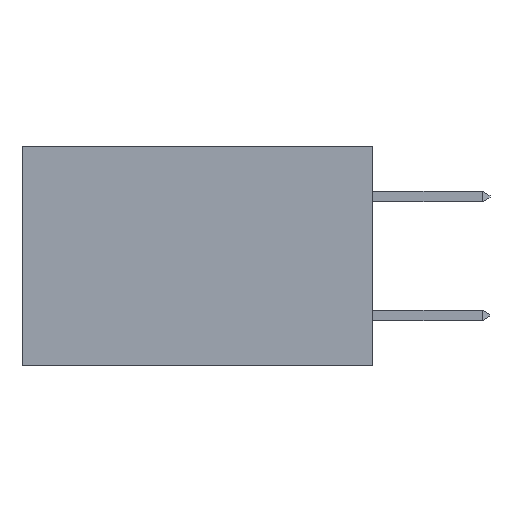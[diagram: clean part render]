
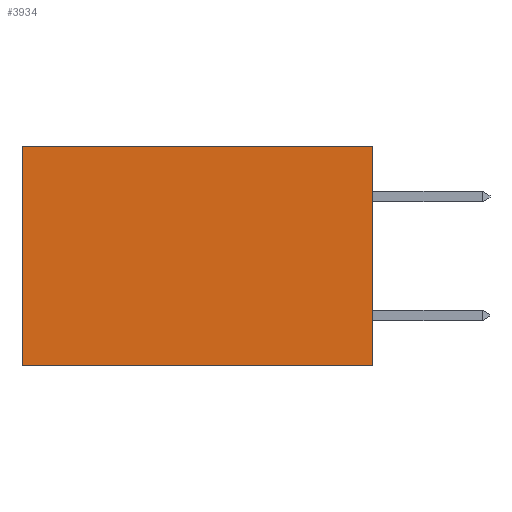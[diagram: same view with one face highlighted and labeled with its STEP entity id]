
A CAD part, left-side view. The second image highlights one B-rep face of the part: STEP entity #3934.
In plain terms, the highlighted planar face has unit normal (-1, 0, 0).
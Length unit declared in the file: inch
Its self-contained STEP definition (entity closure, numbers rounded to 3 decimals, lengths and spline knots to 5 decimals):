
#102 = ORIENTED_EDGE ( 'NONE', *, *, #2369, .F. ) ;
#112 = ORIENTED_EDGE ( 'NONE', *, *, #5296, .F. ) ;
#225 = CARTESIAN_POINT ( 'NONE',  ( 0.277, 0., 0. ) ) ;
#416 = DIRECTION ( 'NONE',  ( 0., 0., -1. ) ) ;
#442 = DIRECTION ( 'NONE',  ( 1., 0., 0. ) ) ;
#554 = CARTESIAN_POINT ( 'NONE',  ( 0.277, 0., -0.37 ) ) ;
#694 = EDGE_CURVE ( 'NONE', #3943, #6967, #5586, .T. ) ;
#910 = VERTEX_POINT ( 'NONE', #6572 ) ;
#919 = AXIS2_PLACEMENT_3D ( 'NONE', #554, #442, #416 ) ;
#962 = PLANE ( 'NONE',  #919 ) ;
#1032 = LINE ( 'NONE', #5519, #7045 ) ;
#1482 = CARTESIAN_POINT ( 'NONE',  ( 0.277, 0., 0. ) ) ;
#1960 = CARTESIAN_POINT ( 'NONE',  ( 0.277, 0., -0.37 ) ) ;
#2357 = CARTESIAN_POINT ( 'NONE',  ( 0.277, 0.59, -0.37 ) ) ;
#2369 = EDGE_CURVE ( 'NONE', #3943, #2423, #5488, .T. ) ;
#2423 = VERTEX_POINT ( 'NONE', #2829 ) ;
#2829 = CARTESIAN_POINT ( 'NONE',  ( 0.277, 0., -0.37 ) ) ;
#3053 = DIRECTION ( 'NONE',  ( 0., 0., -1. ) ) ;
#3250 = DIRECTION ( 'NONE',  ( 0., 0., -1. ) ) ;
#3637 = EDGE_LOOP ( 'NONE', ( #4328, #112, #102, #5373 ) ) ;
#3934 = ADVANCED_FACE ( 'NONE', ( #5837 ), #962, .F. ) ;
#3943 = VERTEX_POINT ( 'NONE', #225 ) ;
#4198 = VECTOR ( 'NONE', #5311, 39.37008 ) ;
#4328 = ORIENTED_EDGE ( 'NONE', *, *, #6259, .T. ) ;
#5296 = EDGE_CURVE ( 'NONE', #2423, #910, #1032, .T. ) ;
#5311 = DIRECTION ( 'NONE',  ( 0., 1., 0. ) ) ;
#5373 = ORIENTED_EDGE ( 'NONE', *, *, #694, .T. ) ;
#5386 = VECTOR ( 'NONE', #3053, 39.37008 ) ;
#5439 = DIRECTION ( 'NONE',  ( 0., 1., 0. ) ) ;
#5488 = LINE ( 'NONE', #1960, #6589 ) ;
#5519 = CARTESIAN_POINT ( 'NONE',  ( 0.277, 0., -0.37 ) ) ;
#5586 = LINE ( 'NONE', #1482, #4198 ) ;
#5837 = FACE_OUTER_BOUND ( 'NONE', #3637, .T. ) ;
#5853 = CARTESIAN_POINT ( 'NONE',  ( 0.277, 0.59, 0. ) ) ;
#6259 = EDGE_CURVE ( 'NONE', #6967, #910, #6624, .T. ) ;
#6572 = CARTESIAN_POINT ( 'NONE',  ( 0.277, 0.59, -0.37 ) ) ;
#6589 = VECTOR ( 'NONE', #3250, 39.37008 ) ;
#6624 = LINE ( 'NONE', #2357, #5386 ) ;
#6967 = VERTEX_POINT ( 'NONE', #5853 ) ;
#7045 = VECTOR ( 'NONE', #5439, 39.37008 ) ;
